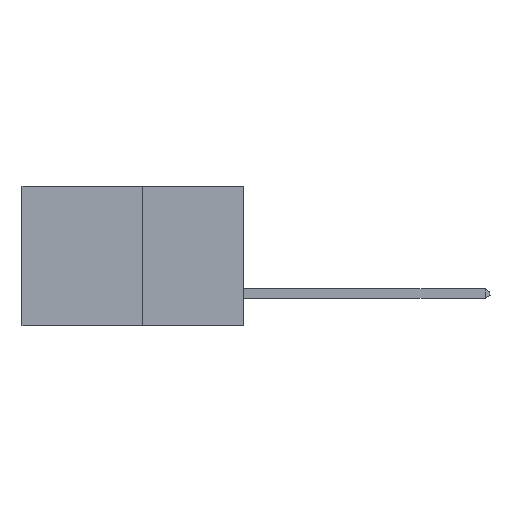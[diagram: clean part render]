
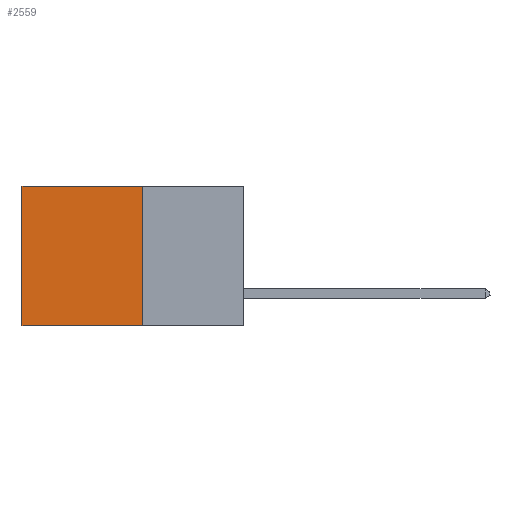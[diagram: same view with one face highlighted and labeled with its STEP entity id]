
A CAD part, left-side view. The second image highlights one B-rep face of the part: STEP entity #2559.
In plain terms, the highlighted planar face has unit normal (-1, 0, 0).
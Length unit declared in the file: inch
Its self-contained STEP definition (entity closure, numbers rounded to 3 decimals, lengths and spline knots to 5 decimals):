
#646 = DIRECTION ( 'NONE',  ( 0., 1., 0. ) ) ;
#2559 = ADVANCED_FACE ( 'NONE', ( #4006 ), #3473, .F. ) ;
#3473 = PLANE ( 'NONE',  #17262 ) ;
#3575 = EDGE_CURVE ( 'NONE', #11702, #14224, #16598, .T. ) ;
#3816 = LINE ( 'NONE', #17398, #14593 ) ;
#4006 = FACE_OUTER_BOUND ( 'NONE', #16468, .T. ) ;
#4606 = CARTESIAN_POINT ( 'NONE',  ( 0.277, 0.59, -0.37 ) ) ;
#4649 = CARTESIAN_POINT ( 'NONE',  ( 0.277, 0.27, -0.37 ) ) ;
#5333 = VERTEX_POINT ( 'NONE', #4606 ) ;
#5558 = VECTOR ( 'NONE', #12169, 39.37008 ) ;
#6875 = CARTESIAN_POINT ( 'NONE',  ( 0.277, 0.59, 0. ) ) ;
#8329 = CARTESIAN_POINT ( 'NONE',  ( 0.277, 0.59, -0.37 ) ) ;
#8575 = VECTOR ( 'NONE', #11986, 39.37008 ) ;
#8639 = CARTESIAN_POINT ( 'NONE',  ( 0.277, 0.27, 0. ) ) ;
#9352 = CARTESIAN_POINT ( 'NONE',  ( 0.277, 0.27, -0.37 ) ) ;
#9604 = EDGE_CURVE ( 'NONE', #11702, #18040, #14019, .T. ) ;
#9741 = DIRECTION ( 'NONE',  ( 0., 0., -1. ) ) ;
#10422 = ORIENTED_EDGE ( 'NONE', *, *, #15668, .T. ) ;
#10467 = ORIENTED_EDGE ( 'NONE', *, *, #14565, .F. ) ;
#11702 = VERTEX_POINT ( 'NONE', #8639 ) ;
#11986 = DIRECTION ( 'NONE',  ( 0., 0., -1. ) ) ;
#12169 = DIRECTION ( 'NONE',  ( 0., 1., 0. ) ) ;
#12331 = CARTESIAN_POINT ( 'NONE',  ( 0.277, 0.27, 0. ) ) ;
#12942 = ORIENTED_EDGE ( 'NONE', *, *, #3575, .T. ) ;
#13901 = VECTOR ( 'NONE', #9741, 39.37008 ) ;
#14019 = LINE ( 'NONE', #17386, #8575 ) ;
#14224 = VERTEX_POINT ( 'NONE', #6875 ) ;
#14565 = EDGE_CURVE ( 'NONE', #18040, #5333, #3816, .T. ) ;
#14593 = VECTOR ( 'NONE', #646, 39.37008 ) ;
#15668 = EDGE_CURVE ( 'NONE', #14224, #5333, #17876, .T. ) ;
#15675 = ORIENTED_EDGE ( 'NONE', *, *, #9604, .F. ) ;
#16468 = EDGE_LOOP ( 'NONE', ( #10422, #10467, #15675, #12942 ) ) ;
#16598 = LINE ( 'NONE', #12331, #5558 ) ;
#17262 = AXIS2_PLACEMENT_3D ( 'NONE', #9352, #17940, #17903 ) ;
#17386 = CARTESIAN_POINT ( 'NONE',  ( 0.277, 0.27, -0.37 ) ) ;
#17398 = CARTESIAN_POINT ( 'NONE',  ( 0.277, 0.27, -0.37 ) ) ;
#17876 = LINE ( 'NONE', #8329, #13901 ) ;
#17903 = DIRECTION ( 'NONE',  ( 0., 0., -1. ) ) ;
#17940 = DIRECTION ( 'NONE',  ( 1., 0., 0. ) ) ;
#18040 = VERTEX_POINT ( 'NONE', #4649 ) ;
